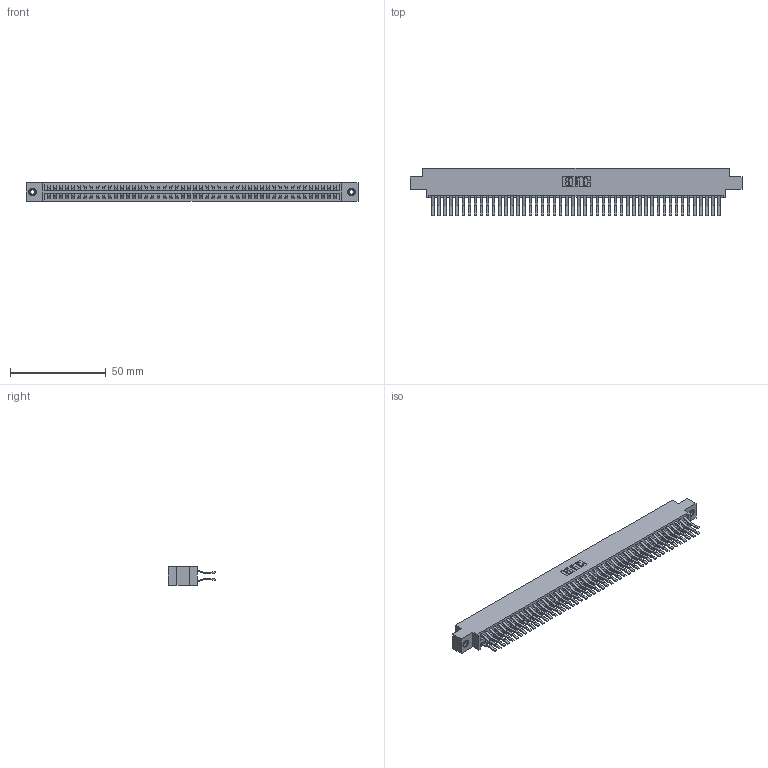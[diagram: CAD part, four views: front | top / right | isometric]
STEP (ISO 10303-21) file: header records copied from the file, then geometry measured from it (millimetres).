
FILE_DESCRIPTION (( 'STEP AP203' ), '1' );
FILE_NAME ('346-096-560-808.STEP', '2018-08-30T08:02:23', ( '' ), ( '' ), 'SwSTEP 2.0', 'SolidWorks 2016', '' );
FILE_SCHEMA (( 'CONFIG_CONTROL_DESIGN' ));
Length unit declared in the file: inch
Products named in the file (4): 345-250-001_345-250-003-102; 346-096-560-808; 346 Part_0.170 Offset - 0.156 Dia-TI; 345-292-001_560 Tail
Assembly tree (99 placements, depth 2):
  346-096-560-808
    346 Part_0.170 Offset - 0.156 Dia-TI
    345-292-001_560 Tail  x96
    345-250-001_345-250-003-102  x2
Bounding box: 172.97 x 24.78 x 9.4 mm (x, y, z)
Volume: 17381.8 mm3; surface area: 25865.2 mm2
Topology: 99 solids, 99 shells, 5370 faces, 15933 edges, 10486 vertices
Faces by surface type: plane 3472, cylinder 1882, cone 12, torus 4
Entity records: 31924 total; most frequent: CARTESIAN_POINT 5239, ORIENTED_EDGE 5166, DIRECTION 4697, EDGE_CURVE 2583, VECTOR 2235, LINE 2235, VERTEX_POINT 1716, AXIS2_PLACEMENT_3D 1231
